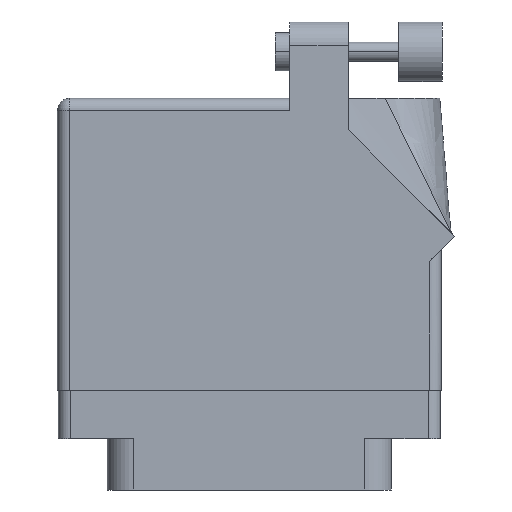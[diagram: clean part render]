
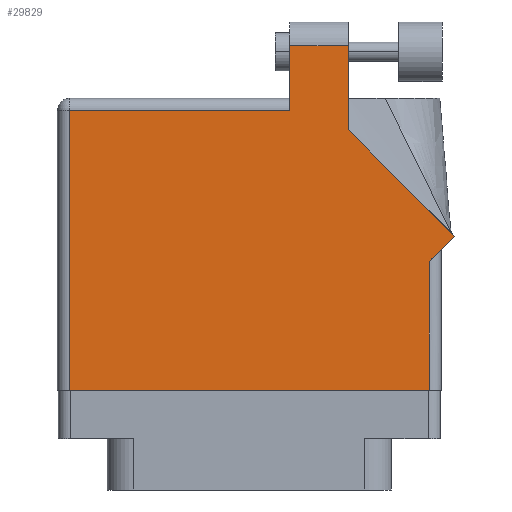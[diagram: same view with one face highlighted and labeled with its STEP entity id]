
A CAD part, front view. The second image highlights one B-rep face of the part: STEP entity #29829.
In plain terms, the highlighted face is planar.
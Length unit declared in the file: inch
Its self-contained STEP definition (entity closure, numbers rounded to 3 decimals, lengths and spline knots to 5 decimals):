
#13 = ORIENTED_EDGE ( 'NONE', *, *, #33514, .T. ) ;
#173 = CARTESIAN_POINT ( 'NONE',  ( -0.943, -0.1, 0.455 ) ) ;
#444 = EDGE_CURVE ( 'NONE', #28140, #27518, #29955, .T. ) ;
#522 = CARTESIAN_POINT ( 'NONE',  ( 0.519, 1.26442, 0.455 ) ) ;
#1762 = CARTESIAN_POINT ( 'NONE',  ( -1.005, -0.1, 0.455 ) ) ;
#1915 = VERTEX_POINT ( 'NONE', #26689 ) ;
#2235 = CARTESIAN_POINT ( 'NONE',  ( -0.943, 1.368, 0.455 ) ) ;
#3005 = DIRECTION ( 'NONE',  ( -1., 0., 0. ) ) ;
#3022 = VERTEX_POINT ( 'NONE', #13036 ) ;
#3882 = CARTESIAN_POINT ( 'NONE',  ( 0.519, 1.705, 0.455 ) ) ;
#4719 = ORIENTED_EDGE ( 'NONE', *, *, #22780, .T. ) ;
#6851 = CARTESIAN_POINT ( 'NONE',  ( 0.212, 1.368, 0.455 ) ) ;
#6944 = ORIENTED_EDGE ( 'NONE', *, *, #22248, .T. ) ;
#7260 = EDGE_CURVE ( 'NONE', #36043, #3022, #9944, .T. ) ;
#7466 = CARTESIAN_POINT ( 'NONE',  ( -0.943, -0.1, 0.455 ) ) ;
#7866 = CARTESIAN_POINT ( 'NONE',  ( 1.07571, 0.70771, 0.455 ) ) ;
#8210 = LINE ( 'NONE', #522, #29551 ) ;
#8701 = LINE ( 'NONE', #35989, #27403 ) ;
#8713 = EDGE_CURVE ( 'NONE', #27518, #35342, #35590, .T. ) ;
#8963 = PLANE ( 'NONE',  #13205 ) ;
#9944 = LINE ( 'NONE', #1762, #20424 ) ;
#10069 = VECTOR ( 'NONE', #19428, 39.37008 ) ;
#10289 = ORIENTED_EDGE ( 'NONE', *, *, #8713, .T. ) ;
#10322 = DIRECTION ( 'NONE',  ( 0., -1., 0. ) ) ;
#10732 = VECTOR ( 'NONE', #3005, 39.37008 ) ;
#11413 = EDGE_CURVE ( 'NONE', #35342, #36043, #17796, .T. ) ;
#11685 = VECTOR ( 'NONE', #16658, 39.37008 ) ;
#12010 = CARTESIAN_POINT ( 'NONE',  ( 0.519, 1.26442, 0.455 ) ) ;
#12096 = CARTESIAN_POINT ( 'NONE',  ( 1.07571, 0.70771, 0.455 ) ) ;
#12833 = CARTESIAN_POINT ( 'NONE',  ( 0.212, 1.705, 0.455 ) ) ;
#13036 = CARTESIAN_POINT ( 'NONE',  ( 0.943, -0.1, 0.455 ) ) ;
#13205 = AXIS2_PLACEMENT_3D ( 'NONE', #28200, #17082, #17214 ) ;
#13275 = ORIENTED_EDGE ( 'NONE', *, *, #7260, .T. ) ;
#13883 = VERTEX_POINT ( 'NONE', #3882 ) ;
#14664 = ORIENTED_EDGE ( 'NONE', *, *, #444, .T. ) ;
#15249 = DIRECTION ( 'NONE',  ( -0.707, 0.707, 0. ) ) ;
#15527 = EDGE_CURVE ( 'NONE', #13883, #28140, #34052, .T. ) ;
#16472 = VECTOR ( 'NONE', #30806, 39.37008 ) ;
#16658 = DIRECTION ( 'NONE',  ( 0., 1., 0. ) ) ;
#17082 = DIRECTION ( 'NONE',  ( 0., 0., -1. ) ) ;
#17214 = DIRECTION ( 'NONE',  ( -1., 0., 0. ) ) ;
#17796 = LINE ( 'NONE', #173, #16472 ) ;
#18003 = VECTOR ( 'NONE', #15249, 39.37008 ) ;
#18994 = CARTESIAN_POINT ( 'NONE',  ( 0.943, 0.637, 0.455 ) ) ;
#19126 = LINE ( 'NONE', #18994, #11685 ) ;
#19372 = ORIENTED_EDGE ( 'NONE', *, *, #27074, .T. ) ;
#19428 = DIRECTION ( 'NONE',  ( -1., 0., 0. ) ) ;
#19549 = DIRECTION ( 'NONE',  ( 0.707, 0.707, 0. ) ) ;
#19935 = DIRECTION ( 'NONE',  ( 0., 1., 0. ) ) ;
#20008 = EDGE_LOOP ( 'NONE', ( #4719, #35259, #14664, #10289, #25047, #13275, #6944, #13, #19372 ) ) ;
#20424 = VECTOR ( 'NONE', #21152, 39.37008 ) ;
#20640 = VERTEX_POINT ( 'NONE', #12010 ) ;
#21152 = DIRECTION ( 'NONE',  ( 1., 0., 0. ) ) ;
#22248 = EDGE_CURVE ( 'NONE', #3022, #1915, #19126, .T. ) ;
#22479 = CARTESIAN_POINT ( 'NONE',  ( 0.212, 1.705, 0.455 ) ) ;
#22780 = EDGE_CURVE ( 'NONE', #20640, #13883, #8210, .T. ) ;
#22895 = CARTESIAN_POINT ( 'NONE',  ( -1.005, 1.368, 0.455 ) ) ;
#23351 = VECTOR ( 'NONE', #10322, 39.37008 ) ;
#25047 = ORIENTED_EDGE ( 'NONE', *, *, #11413, .T. ) ;
#25435 = LINE ( 'NONE', #12096, #18003 ) ;
#26689 = CARTESIAN_POINT ( 'NONE',  ( 0.943, 0.575, 0.455 ) ) ;
#27074 = EDGE_CURVE ( 'NONE', #29266, #20640, #25435, .T. ) ;
#27403 = VECTOR ( 'NONE', #19549, 39.37008 ) ;
#27518 = VERTEX_POINT ( 'NONE', #6851 ) ;
#28140 = VERTEX_POINT ( 'NONE', #12833 ) ;
#28200 = CARTESIAN_POINT ( 'NONE',  ( -1.005, 1.43, 0.455 ) ) ;
#29266 = VERTEX_POINT ( 'NONE', #7866 ) ;
#29551 = VECTOR ( 'NONE', #19935, 39.37008 ) ;
#29829 = ADVANCED_FACE ( 'NONE', ( #35687 ), #8963, .F. ) ;
#29955 = LINE ( 'NONE', #35530, #23351 ) ;
#30806 = DIRECTION ( 'NONE',  ( 0., -1., 0. ) ) ;
#33514 = EDGE_CURVE ( 'NONE', #1915, #29266, #8701, .T. ) ;
#34052 = LINE ( 'NONE', #22479, #10069 ) ;
#35259 = ORIENTED_EDGE ( 'NONE', *, *, #15527, .T. ) ;
#35342 = VERTEX_POINT ( 'NONE', #2235 ) ;
#35530 = CARTESIAN_POINT ( 'NONE',  ( 0.212, 1.43, 0.455 ) ) ;
#35590 = LINE ( 'NONE', #22895, #10732 ) ;
#35687 = FACE_OUTER_BOUND ( 'NONE', #20008, .T. ) ;
#35989 = CARTESIAN_POINT ( 'NONE',  ( 1.005, 0.637, 0.455 ) ) ;
#36043 = VERTEX_POINT ( 'NONE', #7466 ) ;
